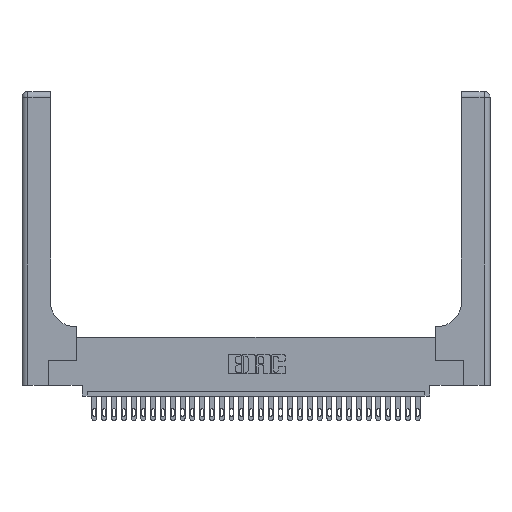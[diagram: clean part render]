
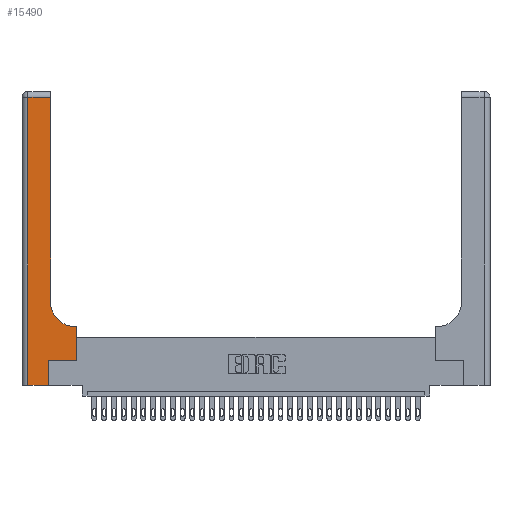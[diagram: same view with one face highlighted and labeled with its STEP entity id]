
A CAD part, top view. The second image highlights one B-rep face of the part: STEP entity #15490.
In plain terms, the highlighted planar face has unit normal (0, 0, 1).
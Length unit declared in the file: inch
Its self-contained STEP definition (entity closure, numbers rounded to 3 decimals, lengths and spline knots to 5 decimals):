
#316 = ORIENTED_EDGE ( 'NONE', *, *, #20299, .T. ) ;
#457 = VECTOR ( 'NONE', #19227, 39.37008 ) ;
#920 = CARTESIAN_POINT ( 'NONE',  ( 0.5415, 0.6, 0.37 ) ) ;
#1193 = DIRECTION ( 'NONE',  ( -1., 0., 0. ) ) ;
#1199 = ORIENTED_EDGE ( 'NONE', *, *, #28155, .T. ) ;
#1538 = EDGE_CURVE ( 'NONE', #17366, #21432, #15716, .T. ) ;
#1589 = CIRCLE ( 'NONE', #10740, 0.25 ) ;
#2276 = VERTEX_POINT ( 'NONE', #21814 ) ;
#2796 = VECTOR ( 'NONE', #5758, 39.37008 ) ;
#2910 = ORIENTED_EDGE ( 'NONE', *, *, #26462, .T. ) ;
#3441 = LINE ( 'NONE', #28356, #21989 ) ;
#3537 = DIRECTION ( 'NONE',  ( 0., 0., -1. ) ) ;
#3816 = VECTOR ( 'NONE', #22803, 39.37008 ) ;
#4214 = LINE ( 'NONE', #10609, #3816 ) ;
#5758 = DIRECTION ( 'NONE',  ( 0., -1., 0. ) ) ;
#5949 = EDGE_CURVE ( 'NONE', #17273, #23603, #16734, .T. ) ;
#5954 = ORIENTED_EDGE ( 'NONE', *, *, #30576, .T. ) ;
#6544 = EDGE_LOOP ( 'NONE', ( #1199, #20640, #2910, #7758, #316, #13501, #20428, #29295, #5954 ) ) ;
#7758 = ORIENTED_EDGE ( 'NONE', *, *, #1538, .T. ) ;
#8621 = AXIS2_PLACEMENT_3D ( 'NONE', #30130, #3537, #1193 ) ;
#8717 = PLANE ( 'NONE',  #8621 ) ;
#9176 = VECTOR ( 'NONE', #21572, 39.37008 ) ;
#9375 = LINE ( 'NONE', #15576, #2796 ) ;
#9942 = CARTESIAN_POINT ( 'NONE',  ( 0.2915, 2.94, 0.37 ) ) ;
#10061 = CARTESIAN_POINT ( 'NONE',  ( 0.269, 0.25, 0.37 ) ) ;
#10609 = CARTESIAN_POINT ( 'NONE',  ( 0.2915, 3., 0.37 ) ) ;
#10740 = AXIS2_PLACEMENT_3D ( 'NONE', #11195, #23671, #23356 ) ;
#11195 = CARTESIAN_POINT ( 'NONE',  ( 0.5415, 0.85, 0.37 ) ) ;
#11432 = CARTESIAN_POINT ( 'NONE',  ( 0.5585, 0.6, 0.37 ) ) ;
#11499 = VECTOR ( 'NONE', #22704, 39.37008 ) ;
#11644 = CARTESIAN_POINT ( 'NONE',  ( 0., 0., 0.37 ) ) ;
#12732 = VECTOR ( 'NONE', #24669, 39.37008 ) ;
#13501 = ORIENTED_EDGE ( 'NONE', *, *, #27595, .T. ) ;
#13878 = VERTEX_POINT ( 'NONE', #28261 ) ;
#14534 = CARTESIAN_POINT ( 'NONE',  ( 0.06, 2.94, 0.37 ) ) ;
#15002 = VERTEX_POINT ( 'NONE', #11432 ) ;
#15490 = ADVANCED_FACE ( 'NONE', ( #30032 ), #8717, .F. ) ;
#15576 = CARTESIAN_POINT ( 'NONE',  ( 0.06, 3., 0.37 ) ) ;
#15716 = LINE ( 'NONE', #11644, #9176 ) ;
#16734 = LINE ( 'NONE', #28156, #18258 ) ;
#17258 = LINE ( 'NONE', #17940, #11499 ) ;
#17273 = VERTEX_POINT ( 'NONE', #9942 ) ;
#17338 = VERTEX_POINT ( 'NONE', #10061 ) ;
#17366 = VERTEX_POINT ( 'NONE', #24822 ) ;
#17940 = CARTESIAN_POINT ( 'NONE',  ( 0.5585, 0.25, 0.37 ) ) ;
#17942 = DIRECTION ( 'NONE',  ( -1., 0., 0. ) ) ;
#18258 = VECTOR ( 'NONE', #17942, 39.37008 ) ;
#18551 = DIRECTION ( 'NONE',  ( 0., 1., 0. ) ) ;
#19227 = DIRECTION ( 'NONE',  ( -1., 0., 0. ) ) ;
#20299 = EDGE_CURVE ( 'NONE', #21432, #17338, #3441, .T. ) ;
#20428 = ORIENTED_EDGE ( 'NONE', *, *, #21253, .T. ) ;
#20640 = ORIENTED_EDGE ( 'NONE', *, *, #5949, .T. ) ;
#20828 = LINE ( 'NONE', #29529, #12732 ) ;
#21253 = EDGE_CURVE ( 'NONE', #13878, #15002, #17258, .T. ) ;
#21408 = CARTESIAN_POINT ( 'NONE',  ( 0.2915, 0.6, 0.37 ) ) ;
#21432 = VERTEX_POINT ( 'NONE', #31324 ) ;
#21572 = DIRECTION ( 'NONE',  ( 1., 0., 0. ) ) ;
#21814 = CARTESIAN_POINT ( 'NONE',  ( 0.2915, 0.85, 0.37 ) ) ;
#21989 = VECTOR ( 'NONE', #18551, 39.37008 ) ;
#22704 = DIRECTION ( 'NONE',  ( 0., 1., 0. ) ) ;
#22803 = DIRECTION ( 'NONE',  ( 0., 1., 0. ) ) ;
#23356 = DIRECTION ( 'NONE',  ( 1., 0., 0. ) ) ;
#23603 = VERTEX_POINT ( 'NONE', #14534 ) ;
#23671 = DIRECTION ( 'NONE',  ( 0., 0., -1. ) ) ;
#24669 = DIRECTION ( 'NONE',  ( 1., 0., 0. ) ) ;
#24822 = CARTESIAN_POINT ( 'NONE',  ( 0.06, 0., 0.37 ) ) ;
#26462 = EDGE_CURVE ( 'NONE', #23603, #17366, #9375, .T. ) ;
#27595 = EDGE_CURVE ( 'NONE', #17338, #13878, #20828, .T. ) ;
#28155 = EDGE_CURVE ( 'NONE', #2276, #17273, #4214, .T. ) ;
#28156 = CARTESIAN_POINT ( 'NONE',  ( 0., 2.94, 0.37 ) ) ;
#28261 = CARTESIAN_POINT ( 'NONE',  ( 0.5585, 0.25, 0.37 ) ) ;
#28356 = CARTESIAN_POINT ( 'NONE',  ( 0.269, 0., 0.37 ) ) ;
#29124 = VERTEX_POINT ( 'NONE', #920 ) ;
#29295 = ORIENTED_EDGE ( 'NONE', *, *, #29452, .T. ) ;
#29452 = EDGE_CURVE ( 'NONE', #15002, #29124, #30111, .T. ) ;
#29529 = CARTESIAN_POINT ( 'NONE',  ( 0.269, 0.25, 0.37 ) ) ;
#30032 = FACE_OUTER_BOUND ( 'NONE', #6544, .T. ) ;
#30111 = LINE ( 'NONE', #21408, #457 ) ;
#30130 = CARTESIAN_POINT ( 'NONE',  ( 0., 3., 0.37 ) ) ;
#30576 = EDGE_CURVE ( 'NONE', #29124, #2276, #1589, .T. ) ;
#31324 = CARTESIAN_POINT ( 'NONE',  ( 0.269, 0., 0.37 ) ) ;
